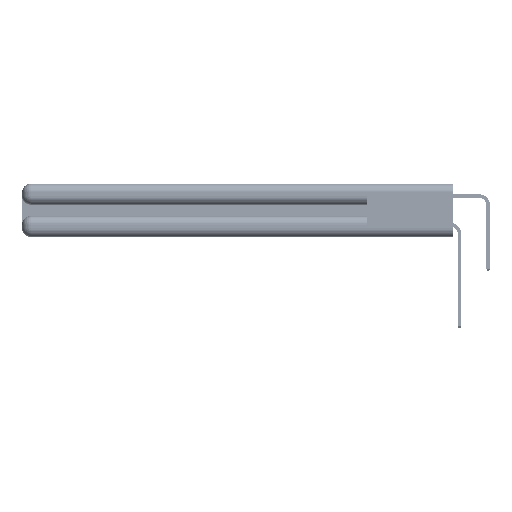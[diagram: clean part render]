
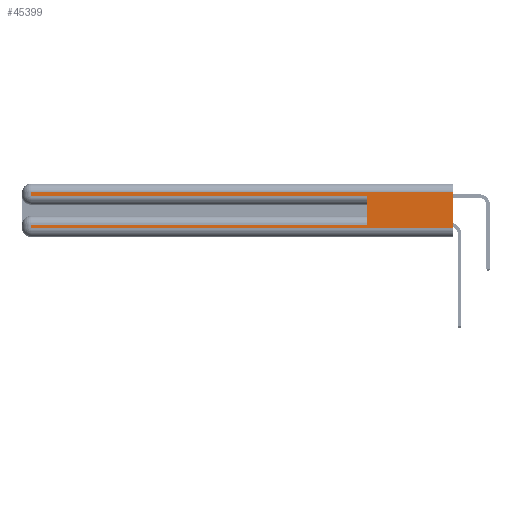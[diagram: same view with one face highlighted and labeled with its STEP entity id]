
A CAD part, left-side view. The second image highlights one B-rep face of the part: STEP entity #45399.
In plain terms, the highlighted planar face has unit normal (-1, 0, 0).
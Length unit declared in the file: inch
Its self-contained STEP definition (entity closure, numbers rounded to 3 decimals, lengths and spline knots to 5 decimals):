
#1013 = CARTESIAN_POINT ( 'NONE',  ( 0., 0., 0.31 ) ) ;
#1671 = LINE ( 'NONE', #49523, #13370 ) ;
#2398 = DIRECTION ( 'NONE',  ( 0., -1., 0. ) ) ;
#2456 = VERTEX_POINT ( 'NONE', #9331 ) ;
#2834 = VECTOR ( 'NONE', #41899, 39.37008 ) ;
#3188 = LINE ( 'NONE', #37377, #24079 ) ;
#3717 = ORIENTED_EDGE ( 'NONE', *, *, #20418, .T. ) ;
#3906 = CARTESIAN_POINT ( 'NONE',  ( 0., 0., 0.31 ) ) ;
#5986 = CARTESIAN_POINT ( 'NONE',  ( 0., 0., 0.06 ) ) ;
#7617 = CARTESIAN_POINT ( 'NONE',  ( 0., 2.94, 0.31 ) ) ;
#8581 = VERTEX_POINT ( 'NONE', #15377 ) ;
#9331 = CARTESIAN_POINT ( 'NONE',  ( 0., 2.94, 0.06 ) ) ;
#9466 = CARTESIAN_POINT ( 'NONE',  ( 0., 0.6, 0.145 ) ) ;
#9635 = DIRECTION ( 'NONE',  ( 0., 0., -1. ) ) ;
#11843 = VECTOR ( 'NONE', #30124, 39.37008 ) ;
#13370 = VECTOR ( 'NONE', #14132, 39.37008 ) ;
#13609 = CARTESIAN_POINT ( 'NONE',  ( 0., 0., 0.37 ) ) ;
#14095 = ORIENTED_EDGE ( 'NONE', *, *, #37560, .F. ) ;
#14132 = DIRECTION ( 'NONE',  ( 0., 0., -1. ) ) ;
#14668 = VECTOR ( 'NONE', #40874, 39.37008 ) ;
#15377 = CARTESIAN_POINT ( 'NONE',  ( 0., 2.94, 0.285 ) ) ;
#15906 = PLANE ( 'NONE',  #19043 ) ;
#17170 = FACE_OUTER_BOUND ( 'NONE', #30306, .T. ) ;
#18224 = VECTOR ( 'NONE', #25644, 39.37008 ) ;
#18317 = LINE ( 'NONE', #3906, #42863 ) ;
#19043 = AXIS2_PLACEMENT_3D ( 'NONE', #43380, #47344, #23824 ) ;
#19169 = ORIENTED_EDGE ( 'NONE', *, *, #33305, .T. ) ;
#19940 = VERTEX_POINT ( 'NONE', #41581 ) ;
#19964 = EDGE_CURVE ( 'NONE', #22047, #8581, #1671, .T. ) ;
#20418 = EDGE_CURVE ( 'NONE', #8581, #19940, #21916, .T. ) ;
#20461 = ORIENTED_EDGE ( 'NONE', *, *, #19964, .T. ) ;
#20512 = EDGE_CURVE ( 'NONE', #34319, #2456, #34133, .T. ) ;
#20578 = LINE ( 'NONE', #13609, #50670 ) ;
#20589 = ORIENTED_EDGE ( 'NONE', *, *, #20512, .T. ) ;
#20865 = VERTEX_POINT ( 'NONE', #1013 ) ;
#21052 = VERTEX_POINT ( 'NONE', #5986 ) ;
#21916 = LINE ( 'NONE', #45208, #18224 ) ;
#22047 = VERTEX_POINT ( 'NONE', #7617 ) ;
#22934 = EDGE_CURVE ( 'NONE', #2456, #21052, #3188, .T. ) ;
#23824 = DIRECTION ( 'NONE',  ( 0., 0., -1. ) ) ;
#24079 = VECTOR ( 'NONE', #2398, 39.37008 ) ;
#25466 = EDGE_CURVE ( 'NONE', #26540, #19940, #45999, .T. ) ;
#25644 = DIRECTION ( 'NONE',  ( 0., -1., 0. ) ) ;
#26540 = VERTEX_POINT ( 'NONE', #50399 ) ;
#29699 = ORIENTED_EDGE ( 'NONE', *, *, #30499, .T. ) ;
#30124 = DIRECTION ( 'NONE',  ( 0., 1., 0. ) ) ;
#30272 = CARTESIAN_POINT ( 'NONE',  ( 0., 2.94, 0.085 ) ) ;
#30306 = EDGE_LOOP ( 'NONE', ( #14095, #19169, #20461, #3717, #41943, #29699, #20589, #40611 ) ) ;
#30499 = EDGE_CURVE ( 'NONE', #26540, #34319, #43160, .T. ) ;
#33305 = EDGE_CURVE ( 'NONE', #20865, #22047, #18317, .T. ) ;
#34133 = LINE ( 'NONE', #37943, #2834 ) ;
#34319 = VERTEX_POINT ( 'NONE', #30272 ) ;
#37377 = CARTESIAN_POINT ( 'NONE',  ( 0., 0., 0.06 ) ) ;
#37560 = EDGE_CURVE ( 'NONE', #20865, #21052, #20578, .T. ) ;
#37943 = CARTESIAN_POINT ( 'NONE',  ( 0., 2.94, 0.37 ) ) ;
#39224 = DIRECTION ( 'NONE',  ( 0., 1., 0. ) ) ;
#40611 = ORIENTED_EDGE ( 'NONE', *, *, #22934, .T. ) ;
#40874 = DIRECTION ( 'NONE',  ( 0., 0., 1. ) ) ;
#41581 = CARTESIAN_POINT ( 'NONE',  ( 0., 0.6, 0.285 ) ) ;
#41899 = DIRECTION ( 'NONE',  ( 0., 0., -1. ) ) ;
#41943 = ORIENTED_EDGE ( 'NONE', *, *, #25466, .F. ) ;
#42863 = VECTOR ( 'NONE', #39224, 39.37008 ) ;
#43160 = LINE ( 'NONE', #49682, #11843 ) ;
#43380 = CARTESIAN_POINT ( 'NONE',  ( 0., 0., 0.37 ) ) ;
#45208 = CARTESIAN_POINT ( 'NONE',  ( 0., 0., 0.285 ) ) ;
#45399 = ADVANCED_FACE ( 'NONE', ( #17170 ), #15906, .F. ) ;
#45999 = LINE ( 'NONE', #9466, #14668 ) ;
#47344 = DIRECTION ( 'NONE',  ( 1., 0., 0. ) ) ;
#49523 = CARTESIAN_POINT ( 'NONE',  ( 0., 2.94, 0.37 ) ) ;
#49682 = CARTESIAN_POINT ( 'NONE',  ( 0., 0., 0.085 ) ) ;
#50399 = CARTESIAN_POINT ( 'NONE',  ( 0., 0.6, 0.085 ) ) ;
#50670 = VECTOR ( 'NONE', #9635, 39.37008 ) ;
